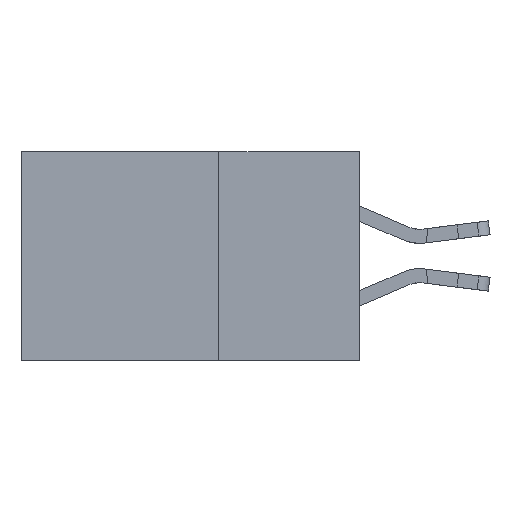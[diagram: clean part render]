
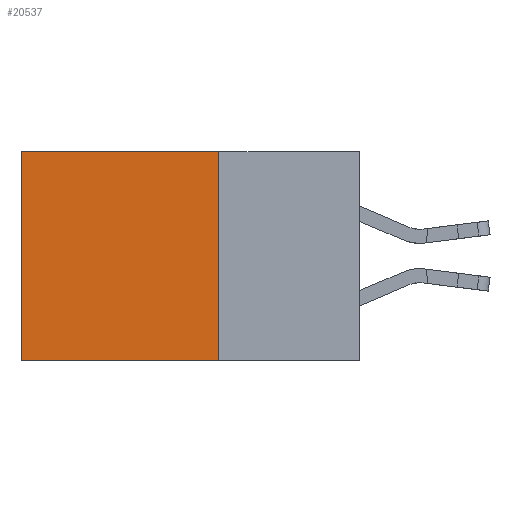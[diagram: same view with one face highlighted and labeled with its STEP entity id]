
A CAD part, left-side view. The second image highlights one B-rep face of the part: STEP entity #20537.
In plain terms, the highlighted planar face has unit normal (-1, 0, 0).
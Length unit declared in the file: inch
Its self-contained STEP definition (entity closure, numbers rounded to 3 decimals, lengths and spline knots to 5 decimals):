
#620 = LINE ( 'NONE', #12646, #15301 ) ;
#1131 = VERTEX_POINT ( 'NONE', #4170 ) ;
#1808 = DIRECTION ( 'NONE',  ( 0., 1., 0. ) ) ;
#2693 = DIRECTION ( 'NONE',  ( 0., 0., -1. ) ) ;
#4170 = CARTESIAN_POINT ( 'NONE',  ( 0.2875, 0.6, -0.37 ) ) ;
#4585 = CARTESIAN_POINT ( 'NONE',  ( 0.2875, 0.25, 0. ) ) ;
#5985 = LINE ( 'NONE', #34569, #30254 ) ;
#6275 = FACE_OUTER_BOUND ( 'NONE', #27099, .T. ) ;
#7989 = VECTOR ( 'NONE', #1808, 39.37008 ) ;
#8065 = DIRECTION ( 'NONE',  ( 1., 0., 0. ) ) ;
#8164 = VECTOR ( 'NONE', #2693, 39.37008 ) ;
#9726 = DIRECTION ( 'NONE',  ( 0., 1., 0. ) ) ;
#10223 = DIRECTION ( 'NONE',  ( 0., 0., -1. ) ) ;
#11364 = ORIENTED_EDGE ( 'NONE', *, *, #24815, .F. ) ;
#12646 = CARTESIAN_POINT ( 'NONE',  ( 0.2875, 0.25, 0. ) ) ;
#14652 = EDGE_CURVE ( 'NONE', #24173, #17696, #620, .T. ) ;
#15301 = VECTOR ( 'NONE', #10223, 39.37008 ) ;
#15693 = VERTEX_POINT ( 'NONE', #17656 ) ;
#15696 = ORIENTED_EDGE ( 'NONE', *, *, #14652, .F. ) ;
#16336 = CARTESIAN_POINT ( 'NONE',  ( 0.2875, 0.6, 0. ) ) ;
#17247 = LINE ( 'NONE', #16336, #8164 ) ;
#17656 = CARTESIAN_POINT ( 'NONE',  ( 0.2875, 0.6, 0. ) ) ;
#17696 = VERTEX_POINT ( 'NONE', #29644 ) ;
#18137 = ORIENTED_EDGE ( 'NONE', *, *, #18725, .T. ) ;
#18725 = EDGE_CURVE ( 'NONE', #24173, #15693, #5985, .T. ) ;
#20537 = ADVANCED_FACE ( 'NONE', ( #6275 ), #24633, .F. ) ;
#22721 = LINE ( 'NONE', #23923, #7989 ) ;
#23604 = ORIENTED_EDGE ( 'NONE', *, *, #35641, .T. ) ;
#23923 = CARTESIAN_POINT ( 'NONE',  ( 0.2875, 0.25, -0.37 ) ) ;
#24173 = VERTEX_POINT ( 'NONE', #4585 ) ;
#24508 = CARTESIAN_POINT ( 'NONE',  ( 0.2875, 0.25, 0. ) ) ;
#24633 = PLANE ( 'NONE',  #27529 ) ;
#24815 = EDGE_CURVE ( 'NONE', #17696, #1131, #22721, .T. ) ;
#27099 = EDGE_LOOP ( 'NONE', ( #23604, #11364, #15696, #18137 ) ) ;
#27529 = AXIS2_PLACEMENT_3D ( 'NONE', #24508, #8065, #35345 ) ;
#29644 = CARTESIAN_POINT ( 'NONE',  ( 0.2875, 0.25, -0.37 ) ) ;
#30254 = VECTOR ( 'NONE', #9726, 39.37008 ) ;
#34569 = CARTESIAN_POINT ( 'NONE',  ( 0.2875, 0.25, 0. ) ) ;
#35345 = DIRECTION ( 'NONE',  ( 0., 0., -1. ) ) ;
#35641 = EDGE_CURVE ( 'NONE', #15693, #1131, #17247, .T. ) ;
